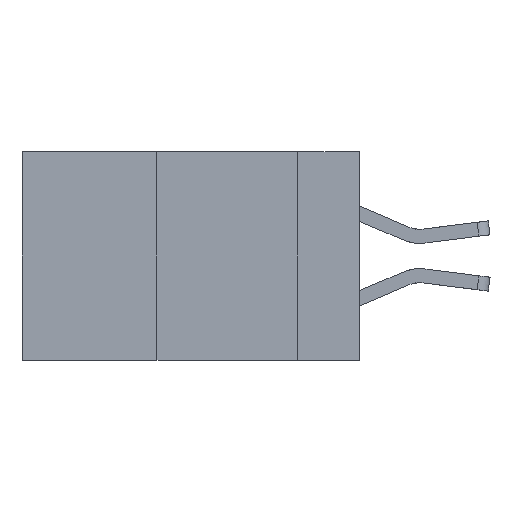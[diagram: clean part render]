
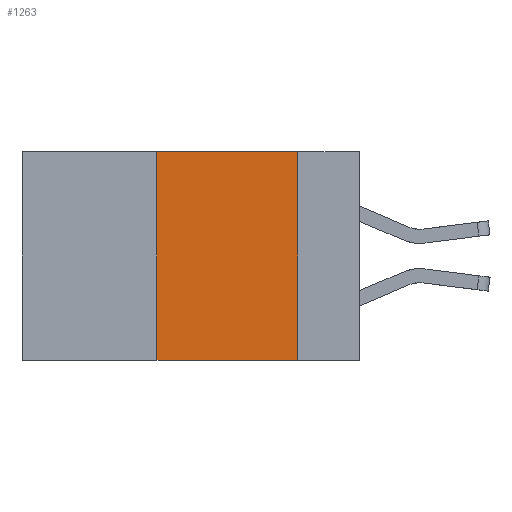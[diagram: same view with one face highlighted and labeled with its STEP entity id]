
A CAD part, left-side view. The second image highlights one B-rep face of the part: STEP entity #1263.
In plain terms, the highlighted planar face has unit normal (-1, 0, 0).
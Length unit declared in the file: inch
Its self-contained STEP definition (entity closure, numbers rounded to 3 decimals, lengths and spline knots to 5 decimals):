
#70 = AXIS2_PLACEMENT_3D ( 'NONE', #4485, #11848, #4540 ) ;
#499 = ORIENTED_EDGE ( 'NONE', *, *, #5667, .F. ) ;
#602 = CARTESIAN_POINT ( 'NONE',  ( 0., 0.11, 0. ) ) ;
#755 = VERTEX_POINT ( 'NONE', #1863 ) ;
#880 = ORIENTED_EDGE ( 'NONE', *, *, #1986, .T. ) ;
#1263 = ADVANCED_FACE ( 'NONE', ( #13356 ), #3297, .F. ) ;
#1400 = CARTESIAN_POINT ( 'NONE',  ( 0., 0.36, 0. ) ) ;
#1842 = VERTEX_POINT ( 'NONE', #602 ) ;
#1863 = CARTESIAN_POINT ( 'NONE',  ( 0., 0.36, -0.37 ) ) ;
#1986 = EDGE_CURVE ( 'NONE', #755, #8840, #6231, .T. ) ;
#2210 = EDGE_CURVE ( 'NONE', #1842, #8840, #13118, .T. ) ;
#2297 = VECTOR ( 'NONE', #14779, 39.37008 ) ;
#2311 = LINE ( 'NONE', #12983, #14476 ) ;
#2633 = VERTEX_POINT ( 'NONE', #5648 ) ;
#2878 = CARTESIAN_POINT ( 'NONE',  ( 0., 0.11, -0.37 ) ) ;
#3297 = PLANE ( 'NONE',  #70 ) ;
#4485 = CARTESIAN_POINT ( 'NONE',  ( 0., 0.6, 0. ) ) ;
#4540 = DIRECTION ( 'NONE',  ( 0., 0., -1. ) ) ;
#5648 = CARTESIAN_POINT ( 'NONE',  ( 0., 0.36, 0. ) ) ;
#5667 = EDGE_CURVE ( 'NONE', #2633, #1842, #2311, .T. ) ;
#6093 = EDGE_CURVE ( 'NONE', #755, #2633, #8855, .T. ) ;
#6231 = LINE ( 'NONE', #15491, #9913 ) ;
#6652 = VECTOR ( 'NONE', #11028, 39.37008 ) ;
#7072 = EDGE_LOOP ( 'NONE', ( #13160, #499, #13523, #880 ) ) ;
#8349 = DIRECTION ( 'NONE',  ( 0., -1., 0. ) ) ;
#8840 = VERTEX_POINT ( 'NONE', #2878 ) ;
#8855 = LINE ( 'NONE', #1400, #2297 ) ;
#9913 = VECTOR ( 'NONE', #8349, 39.37008 ) ;
#11028 = DIRECTION ( 'NONE',  ( 0., 0., -1. ) ) ;
#11848 = DIRECTION ( 'NONE',  ( 1., 0., 0. ) ) ;
#12234 = CARTESIAN_POINT ( 'NONE',  ( 0., 0.11, 0. ) ) ;
#12983 = CARTESIAN_POINT ( 'NONE',  ( 0., 0.6, 0. ) ) ;
#13118 = LINE ( 'NONE', #12234, #6652 ) ;
#13160 = ORIENTED_EDGE ( 'NONE', *, *, #2210, .F. ) ;
#13356 = FACE_OUTER_BOUND ( 'NONE', #7072, .T. ) ;
#13523 = ORIENTED_EDGE ( 'NONE', *, *, #6093, .F. ) ;
#14161 = DIRECTION ( 'NONE',  ( 0., -1., 0. ) ) ;
#14476 = VECTOR ( 'NONE', #14161, 39.37008 ) ;
#14779 = DIRECTION ( 'NONE',  ( 0., 0., 1. ) ) ;
#15491 = CARTESIAN_POINT ( 'NONE',  ( 0., 0.6, -0.37 ) ) ;
